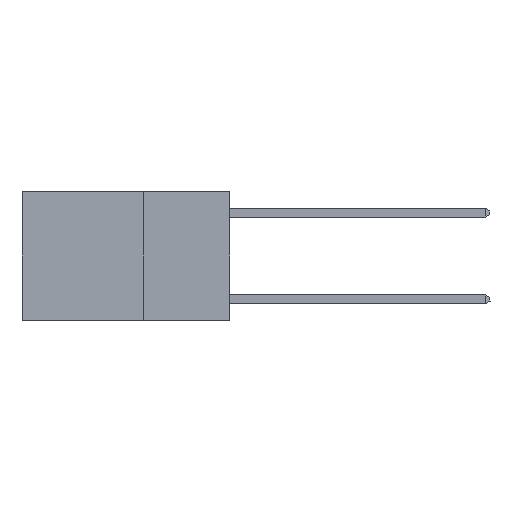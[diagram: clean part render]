
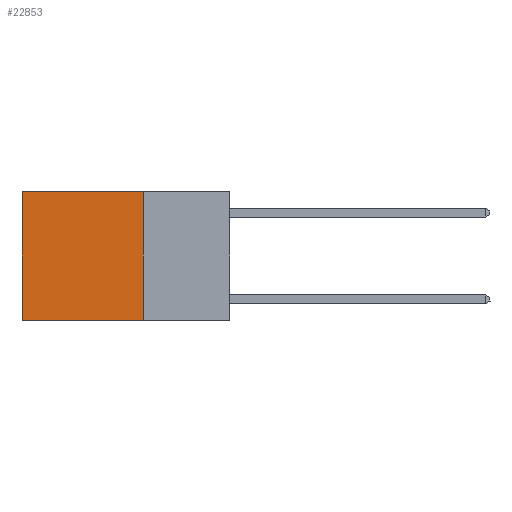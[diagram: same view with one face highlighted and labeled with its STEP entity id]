
A CAD part, left-side view. The second image highlights one B-rep face of the part: STEP entity #22853.
In plain terms, the highlighted planar face has unit normal (-1, 0, 0).
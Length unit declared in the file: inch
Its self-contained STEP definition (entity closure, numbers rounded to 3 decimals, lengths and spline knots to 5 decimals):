
#39 = CARTESIAN_POINT ( 'NONE',  ( 0.2625, 0.25, 0. ) ) ;
#1833 = CARTESIAN_POINT ( 'NONE',  ( 0.2625, 0.25, 0. ) ) ;
#1856 = PLANE ( 'NONE',  #19674 ) ;
#3948 = DIRECTION ( 'NONE',  ( 0., 0., -1. ) ) ;
#4114 = VERTEX_POINT ( 'NONE', #19987 ) ;
#4659 = LINE ( 'NONE', #6579, #14847 ) ;
#5472 = EDGE_CURVE ( 'NONE', #13439, #4114, #20472, .T. ) ;
#5555 = EDGE_CURVE ( 'NONE', #17220, #6973, #22719, .T. ) ;
#6264 = CARTESIAN_POINT ( 'NONE',  ( 0.2625, 0.25, -0.37 ) ) ;
#6579 = CARTESIAN_POINT ( 'NONE',  ( 0.2625, 0.6, 0. ) ) ;
#6973 = VERTEX_POINT ( 'NONE', #17183 ) ;
#7420 = EDGE_CURVE ( 'NONE', #13439, #17220, #10148, .T. ) ;
#8291 = DIRECTION ( 'NONE',  ( 0., 1., 0. ) ) ;
#8620 = DIRECTION ( 'NONE',  ( 0., 0., -1. ) ) ;
#8720 = ORIENTED_EDGE ( 'NONE', *, *, #5555, .F. ) ;
#8844 = EDGE_CURVE ( 'NONE', #4114, #6973, #4659, .T. ) ;
#9922 = CARTESIAN_POINT ( 'NONE',  ( 0.2625, 0.25, 0. ) ) ;
#10063 = CARTESIAN_POINT ( 'NONE',  ( 0.2625, 0.25, 0. ) ) ;
#10148 = LINE ( 'NONE', #39, #20394 ) ;
#13439 = VERTEX_POINT ( 'NONE', #1833 ) ;
#13726 = ORIENTED_EDGE ( 'NONE', *, *, #8844, .T. ) ;
#14496 = EDGE_LOOP ( 'NONE', ( #13726, #8720, #19992, #24711 ) ) ;
#14847 = VECTOR ( 'NONE', #8620, 39.37008 ) ;
#16164 = DIRECTION ( 'NONE',  ( 1., 0., 0. ) ) ;
#17183 = CARTESIAN_POINT ( 'NONE',  ( 0.2625, 0.6, -0.37 ) ) ;
#17220 = VERTEX_POINT ( 'NONE', #18019 ) ;
#17894 = VECTOR ( 'NONE', #8291, 39.37008 ) ;
#18019 = CARTESIAN_POINT ( 'NONE',  ( 0.2625, 0.25, -0.37 ) ) ;
#19674 = AXIS2_PLACEMENT_3D ( 'NONE', #9922, #16164, #3948 ) ;
#19987 = CARTESIAN_POINT ( 'NONE',  ( 0.2625, 0.6, 0. ) ) ;
#19992 = ORIENTED_EDGE ( 'NONE', *, *, #7420, .F. ) ;
#20394 = VECTOR ( 'NONE', #24712, 39.37008 ) ;
#20472 = LINE ( 'NONE', #10063, #24650 ) ;
#22719 = LINE ( 'NONE', #6264, #17894 ) ;
#22853 = ADVANCED_FACE ( 'NONE', ( #26068 ), #1856, .F. ) ;
#24317 = DIRECTION ( 'NONE',  ( 0., 1., 0. ) ) ;
#24650 = VECTOR ( 'NONE', #24317, 39.37008 ) ;
#24711 = ORIENTED_EDGE ( 'NONE', *, *, #5472, .T. ) ;
#24712 = DIRECTION ( 'NONE',  ( 0., 0., -1. ) ) ;
#26068 = FACE_OUTER_BOUND ( 'NONE', #14496, .T. ) ;
